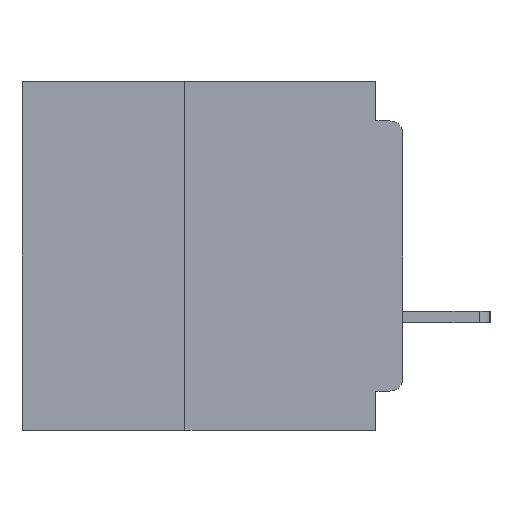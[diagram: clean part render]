
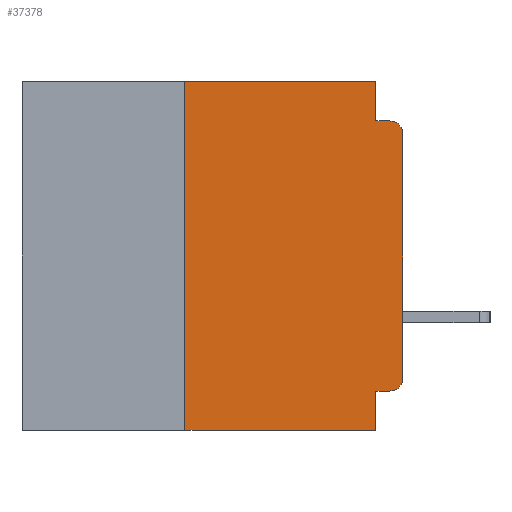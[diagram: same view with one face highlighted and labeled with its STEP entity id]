
A CAD part, left-side view. The second image highlights one B-rep face of the part: STEP entity #37378.
In plain terms, the highlighted planar face has unit normal (-1, 0, 0).
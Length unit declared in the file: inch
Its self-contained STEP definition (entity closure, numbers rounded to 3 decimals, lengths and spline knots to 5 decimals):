
#128 = CARTESIAN_POINT ( 'NONE',  ( 0., 0.437, -0.4 ) ) ;
#130 = DIRECTION ( 'NONE',  ( 0., 0., -1. ) ) ;
#757 = DIRECTION ( 'NONE',  ( 0., -1., 0. ) ) ;
#773 = CARTESIAN_POINT ( 'NONE',  ( 0., 0.25, -0.4 ) ) ;
#999 = DIRECTION ( 'NONE',  ( 0., 0., -1. ) ) ;
#1283 = EDGE_CURVE ( 'NONE', #51401, #23400, #37887, .T. ) ;
#1513 = ORIENTED_EDGE ( 'NONE', *, *, #45285, .F. ) ;
#2236 = LINE ( 'NONE', #4806, #42221 ) ;
#2989 = CARTESIAN_POINT ( 'NONE',  ( 0., 0.031, -0.045 ) ) ;
#3809 = CARTESIAN_POINT ( 'NONE',  ( 0., 0.031, -0.4 ) ) ;
#3914 = CARTESIAN_POINT ( 'NONE',  ( 0., 0.031, -0.4 ) ) ;
#4429 = VERTEX_POINT ( 'NONE', #14059 ) ;
#4806 = CARTESIAN_POINT ( 'NONE',  ( 0., 0., -0.355 ) ) ;
#5978 = EDGE_CURVE ( 'NONE', #20596, #29184, #2236, .T. ) ;
#7148 = VERTEX_POINT ( 'NONE', #3809 ) ;
#7385 = DIRECTION ( 'NONE',  ( 0., 0., 1. ) ) ;
#8052 = ORIENTED_EDGE ( 'NONE', *, *, #39927, .T. ) ;
#8530 = LINE ( 'NONE', #11451, #39087 ) ;
#8765 = CARTESIAN_POINT ( 'NONE',  ( 0., 0.25, 0. ) ) ;
#9537 = LINE ( 'NONE', #3914, #40063 ) ;
#10948 = DIRECTION ( 'NONE',  ( 0., 0., -1. ) ) ;
#11451 = CARTESIAN_POINT ( 'NONE',  ( 0., 0., 0. ) ) ;
#11492 = AXIS2_PLACEMENT_3D ( 'NONE', #45897, #22039, #49900 ) ;
#12901 = DIRECTION ( 'NONE',  ( 0., 1., 0. ) ) ;
#13374 = ORIENTED_EDGE ( 'NONE', *, *, #37254, .F. ) ;
#14059 = CARTESIAN_POINT ( 'NONE',  ( 0., 0.031, 0. ) ) ;
#15609 = CARTESIAN_POINT ( 'NONE',  ( 0., 0.015, -0.355 ) ) ;
#15981 = VERTEX_POINT ( 'NONE', #45779 ) ;
#16167 = ORIENTED_EDGE ( 'NONE', *, *, #49711, .F. ) ;
#17495 = LINE ( 'NONE', #19026, #37422 ) ;
#17575 = EDGE_CURVE ( 'NONE', #4429, #26720, #20077, .T. ) ;
#19026 = CARTESIAN_POINT ( 'NONE',  ( 0., 0.437, 0. ) ) ;
#20047 = DIRECTION ( 'NONE',  ( 0., -1., 0. ) ) ;
#20077 = LINE ( 'NONE', #26799, #29418 ) ;
#20488 = LINE ( 'NONE', #44556, #29828 ) ;
#20596 = VERTEX_POINT ( 'NONE', #15609 ) ;
#20858 = ORIENTED_EDGE ( 'NONE', *, *, #42466, .F. ) ;
#21037 = ORIENTED_EDGE ( 'NONE', *, *, #5978, .F. ) ;
#22039 = DIRECTION ( 'NONE',  ( -1., 0., 0. ) ) ;
#22953 = VECTOR ( 'NONE', #20047, 39.37008 ) ;
#23047 = DIRECTION ( 'NONE',  ( 0., -1., 0. ) ) ;
#23230 = DIRECTION ( 'NONE',  ( -1., 0., 0. ) ) ;
#23400 = VERTEX_POINT ( 'NONE', #48191 ) ;
#24198 = CARTESIAN_POINT ( 'NONE',  ( 0., 0., -0.06 ) ) ;
#24841 = AXIS2_PLACEMENT_3D ( 'NONE', #47085, #23230, #51093 ) ;
#24921 = DIRECTION ( 'NONE',  ( 1., 0., 0. ) ) ;
#26261 = ORIENTED_EDGE ( 'NONE', *, *, #1283, .T. ) ;
#26720 = VERTEX_POINT ( 'NONE', #2989 ) ;
#26799 = CARTESIAN_POINT ( 'NONE',  ( 0., 0.031, 0. ) ) ;
#26882 = VERTEX_POINT ( 'NONE', #44001 ) ;
#28694 = DIRECTION ( 'NONE',  ( 0., 0., 1. ) ) ;
#29026 = EDGE_CURVE ( 'NONE', #20596, #26882, #39161, .T. ) ;
#29184 = VERTEX_POINT ( 'NONE', #43605 ) ;
#29418 = VECTOR ( 'NONE', #10948, 39.37008 ) ;
#29828 = VECTOR ( 'NONE', #757, 39.37008 ) ;
#31201 = EDGE_LOOP ( 'NONE', ( #31854, #26261, #20858, #36727, #16167, #1513, #8052, #13374, #21037, #37960 ) ) ;
#31854 = ORIENTED_EDGE ( 'NONE', *, *, #40455, .T. ) ;
#32565 = FACE_OUTER_BOUND ( 'NONE', #31201, .T. ) ;
#32720 = PLANE ( 'NONE',  #44842 ) ;
#33527 = LINE ( 'NONE', #128, #22953 ) ;
#36727 = ORIENTED_EDGE ( 'NONE', *, *, #17575, .F. ) ;
#37254 = EDGE_CURVE ( 'NONE', #29184, #7148, #9537, .T. ) ;
#37378 = ADVANCED_FACE ( 'NONE', ( #32565 ), #32720, .F. ) ;
#37422 = VECTOR ( 'NONE', #23047, 39.37008 ) ;
#37887 = CIRCLE ( 'NONE', #11492, 0.015 ) ;
#37960 = ORIENTED_EDGE ( 'NONE', *, *, #29026, .T. ) ;
#39087 = VECTOR ( 'NONE', #7385, 39.37008 ) ;
#39161 = CIRCLE ( 'NONE', #24841, 0.015 ) ;
#39927 = EDGE_CURVE ( 'NONE', #15981, #7148, #33527, .T. ) ;
#40063 = VECTOR ( 'NONE', #130, 39.37008 ) ;
#40171 = LINE ( 'NONE', #773, #49524 ) ;
#40455 = EDGE_CURVE ( 'NONE', #26882, #51401, #8530, .T. ) ;
#42221 = VECTOR ( 'NONE', #12901, 39.37008 ) ;
#42466 = EDGE_CURVE ( 'NONE', #26720, #23400, #20488, .T. ) ;
#43605 = CARTESIAN_POINT ( 'NONE',  ( 0., 0.031, -0.355 ) ) ;
#44001 = CARTESIAN_POINT ( 'NONE',  ( 0., 0., -0.34 ) ) ;
#44556 = CARTESIAN_POINT ( 'NONE',  ( 0., 0., -0.045 ) ) ;
#44842 = AXIS2_PLACEMENT_3D ( 'NONE', #48781, #24921, #999 ) ;
#45285 = EDGE_CURVE ( 'NONE', #15981, #49352, #40171, .T. ) ;
#45779 = CARTESIAN_POINT ( 'NONE',  ( 0., 0.25, -0.4 ) ) ;
#45897 = CARTESIAN_POINT ( 'NONE',  ( 0., 0.015, -0.06 ) ) ;
#47085 = CARTESIAN_POINT ( 'NONE',  ( 0., 0.015, -0.34 ) ) ;
#48191 = CARTESIAN_POINT ( 'NONE',  ( 0., 0.015, -0.045 ) ) ;
#48781 = CARTESIAN_POINT ( 'NONE',  ( 0., 0.437, 0. ) ) ;
#49352 = VERTEX_POINT ( 'NONE', #8765 ) ;
#49524 = VECTOR ( 'NONE', #28694, 39.37008 ) ;
#49711 = EDGE_CURVE ( 'NONE', #49352, #4429, #17495, .T. ) ;
#49900 = DIRECTION ( 'NONE',  ( 0., 0., -1. ) ) ;
#51093 = DIRECTION ( 'NONE',  ( 0., 0., -1. ) ) ;
#51401 = VERTEX_POINT ( 'NONE', #24198 ) ;
